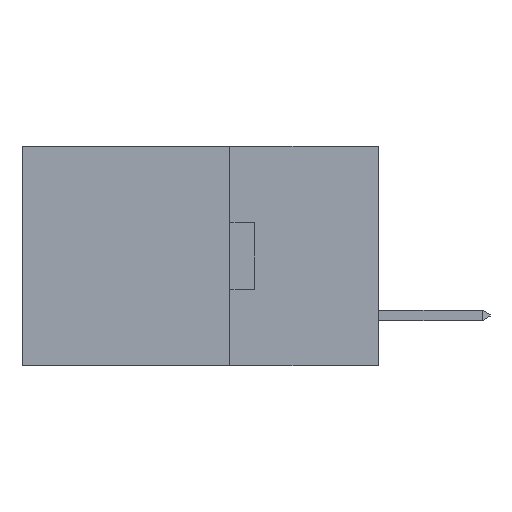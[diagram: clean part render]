
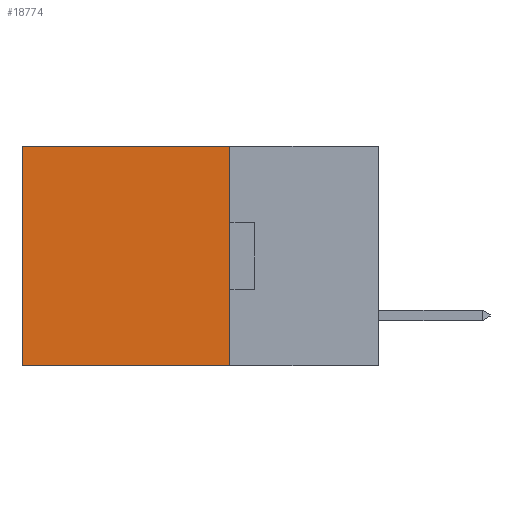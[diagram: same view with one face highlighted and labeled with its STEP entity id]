
A CAD part, left-side view. The second image highlights one B-rep face of the part: STEP entity #18774.
In plain terms, the highlighted planar face has unit normal (-1, 0, 0).
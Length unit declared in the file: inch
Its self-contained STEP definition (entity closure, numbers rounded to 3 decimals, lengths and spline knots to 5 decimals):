
#1301 = DIRECTION ( 'NONE',  ( 0., 0., -1. ) ) ;
#2986 = VERTEX_POINT ( 'NONE', #9542 ) ;
#3134 = EDGE_CURVE ( 'NONE', #25444, #11457, #20838, .T. ) ;
#3672 = AXIS2_PLACEMENT_3D ( 'NONE', #22183, #13956, #1301 ) ;
#3799 = CARTESIAN_POINT ( 'NONE',  ( 0.2615, 0.25, 0. ) ) ;
#3836 = DIRECTION ( 'NONE',  ( 0., 1., 0. ) ) ;
#4024 = DIRECTION ( 'NONE',  ( 0., 0., -1. ) ) ;
#7345 = CARTESIAN_POINT ( 'NONE',  ( 0.2615, 0.25, -0.37 ) ) ;
#9542 = CARTESIAN_POINT ( 'NONE',  ( 0.2615, 0.6, -0.37 ) ) ;
#10302 = CARTESIAN_POINT ( 'NONE',  ( 0.2615, 0.25, -0.37 ) ) ;
#11057 = EDGE_LOOP ( 'NONE', ( #23316, #24695, #18053, #24095 ) ) ;
#11457 = VERTEX_POINT ( 'NONE', #21044 ) ;
#11476 = CARTESIAN_POINT ( 'NONE',  ( 0.2615, 0.25, -0.37 ) ) ;
#11604 = DIRECTION ( 'NONE',  ( 0., 0., -1. ) ) ;
#13005 = VECTOR ( 'NONE', #11604, 39.37008 ) ;
#13211 = EDGE_CURVE ( 'NONE', #11457, #2986, #14937, .T. ) ;
#13956 = DIRECTION ( 'NONE',  ( 1., 0., 0. ) ) ;
#14470 = DIRECTION ( 'NONE',  ( 0., 1., 0. ) ) ;
#14937 = LINE ( 'NONE', #24758, #25199 ) ;
#16567 = FACE_OUTER_BOUND ( 'NONE', #11057, .T. ) ;
#16622 = VECTOR ( 'NONE', #3836, 39.37008 ) ;
#18053 = ORIENTED_EDGE ( 'NONE', *, *, #18677, .F. ) ;
#18575 = VECTOR ( 'NONE', #14470, 39.37008 ) ;
#18677 = EDGE_CURVE ( 'NONE', #25444, #19647, #23954, .T. ) ;
#18774 = ADVANCED_FACE ( 'NONE', ( #16567 ), #26236, .F. ) ;
#19647 = VERTEX_POINT ( 'NONE', #11476 ) ;
#20838 = LINE ( 'NONE', #3799, #16622 ) ;
#21044 = CARTESIAN_POINT ( 'NONE',  ( 0.2615, 0.6, 0. ) ) ;
#21509 = CARTESIAN_POINT ( 'NONE',  ( 0.2615, 0.25, 0. ) ) ;
#22183 = CARTESIAN_POINT ( 'NONE',  ( 0.2615, 0.25, -0.37 ) ) ;
#23316 = ORIENTED_EDGE ( 'NONE', *, *, #13211, .T. ) ;
#23954 = LINE ( 'NONE', #7345, #13005 ) ;
#24014 = LINE ( 'NONE', #10302, #18575 ) ;
#24095 = ORIENTED_EDGE ( 'NONE', *, *, #3134, .T. ) ;
#24653 = EDGE_CURVE ( 'NONE', #19647, #2986, #24014, .T. ) ;
#24695 = ORIENTED_EDGE ( 'NONE', *, *, #24653, .F. ) ;
#24758 = CARTESIAN_POINT ( 'NONE',  ( 0.2615, 0.6, -0.37 ) ) ;
#25199 = VECTOR ( 'NONE', #4024, 39.37008 ) ;
#25444 = VERTEX_POINT ( 'NONE', #21509 ) ;
#26236 = PLANE ( 'NONE',  #3672 ) ;
